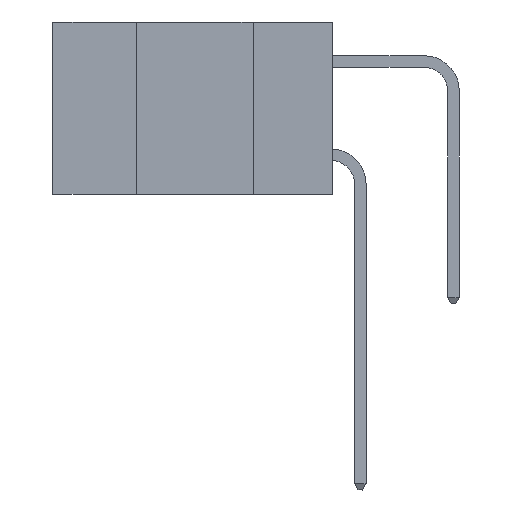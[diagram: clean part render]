
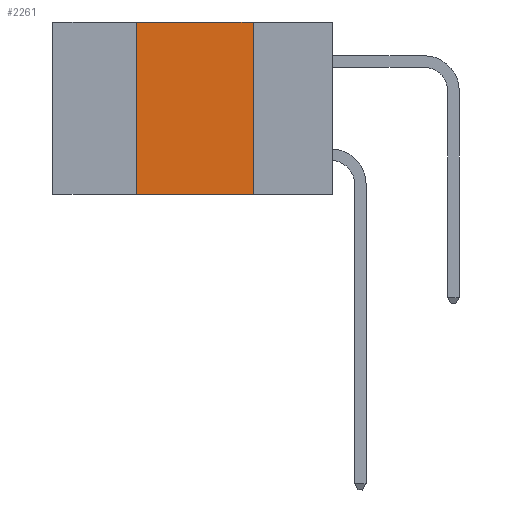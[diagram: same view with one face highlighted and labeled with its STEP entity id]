
A CAD part, left-side view. The second image highlights one B-rep face of the part: STEP entity #2261.
In plain terms, the highlighted planar face has unit normal (-1, 0, 0).
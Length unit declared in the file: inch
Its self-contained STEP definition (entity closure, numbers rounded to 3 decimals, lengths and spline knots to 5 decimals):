
#7 = EDGE_CURVE ( 'NONE', #3152, #10211, #8119, .T. ) ;
#62 = LINE ( 'NONE', #12659, #11770 ) ;
#537 = PLANE ( 'NONE',  #19529 ) ;
#1294 = ORIENTED_EDGE ( 'NONE', *, *, #7, .F. ) ;
#1698 = DIRECTION ( 'NONE',  ( 1., 0., 0. ) ) ;
#1896 = CARTESIAN_POINT ( 'NONE',  ( 0., 0.6, 0. ) ) ;
#2008 = DIRECTION ( 'NONE',  ( 0., -1., 0. ) ) ;
#2261 = ADVANCED_FACE ( 'NONE', ( #4442 ), #537, .F. ) ;
#3152 = VERTEX_POINT ( 'NONE', #18307 ) ;
#3380 = VECTOR ( 'NONE', #13019, 39.37008 ) ;
#3688 = EDGE_LOOP ( 'NONE', ( #12992, #9601, #1294, #14664 ) ) ;
#3842 = EDGE_CURVE ( 'NONE', #3152, #5900, #16061, .T. ) ;
#4442 = FACE_OUTER_BOUND ( 'NONE', #3688, .T. ) ;
#5672 = CARTESIAN_POINT ( 'NONE',  ( 0., 0.6, -0.37 ) ) ;
#5900 = VERTEX_POINT ( 'NONE', #19034 ) ;
#6162 = EDGE_CURVE ( 'NONE', #9309, #5900, #19373, .T. ) ;
#7203 = DIRECTION ( 'NONE',  ( 0., -1., 0. ) ) ;
#7635 = VECTOR ( 'NONE', #12418, 39.37008 ) ;
#8119 = LINE ( 'NONE', #11406, #7635 ) ;
#9309 = VERTEX_POINT ( 'NONE', #10167 ) ;
#9601 = ORIENTED_EDGE ( 'NONE', *, *, #11662, .F. ) ;
#10167 = CARTESIAN_POINT ( 'NONE',  ( 0., 0.17, 0. ) ) ;
#10211 = VERTEX_POINT ( 'NONE', #13773 ) ;
#10659 = DIRECTION ( 'NONE',  ( 0., 0., -1. ) ) ;
#11406 = CARTESIAN_POINT ( 'NONE',  ( 0., 0.42, 0. ) ) ;
#11662 = EDGE_CURVE ( 'NONE', #10211, #9309, #62, .T. ) ;
#11770 = VECTOR ( 'NONE', #2008, 39.37008 ) ;
#12418 = DIRECTION ( 'NONE',  ( 0., 0., 1. ) ) ;
#12659 = CARTESIAN_POINT ( 'NONE',  ( 0., 0.6, 0. ) ) ;
#12992 = ORIENTED_EDGE ( 'NONE', *, *, #6162, .F. ) ;
#13019 = DIRECTION ( 'NONE',  ( 0., 0., -1. ) ) ;
#13152 = CARTESIAN_POINT ( 'NONE',  ( 0., 0.17, 0. ) ) ;
#13773 = CARTESIAN_POINT ( 'NONE',  ( 0., 0.42, 0. ) ) ;
#14664 = ORIENTED_EDGE ( 'NONE', *, *, #3842, .T. ) ;
#16061 = LINE ( 'NONE', #5672, #19481 ) ;
#18307 = CARTESIAN_POINT ( 'NONE',  ( 0., 0.42, -0.37 ) ) ;
#19034 = CARTESIAN_POINT ( 'NONE',  ( 0., 0.17, -0.37 ) ) ;
#19373 = LINE ( 'NONE', #13152, #3380 ) ;
#19481 = VECTOR ( 'NONE', #7203, 39.37008 ) ;
#19529 = AXIS2_PLACEMENT_3D ( 'NONE', #1896, #1698, #10659 ) ;
